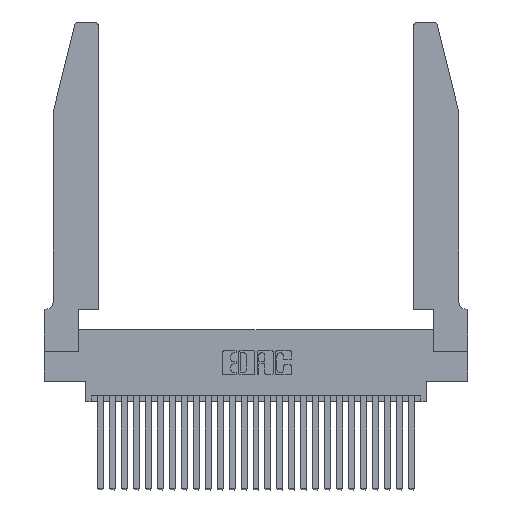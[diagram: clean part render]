
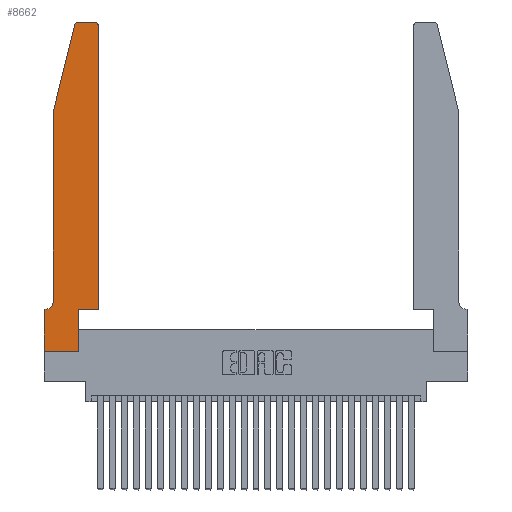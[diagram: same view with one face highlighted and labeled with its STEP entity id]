
A CAD part, top view. The second image highlights one B-rep face of the part: STEP entity #8662.
In plain terms, the highlighted planar face has unit normal (0, 0, 1).
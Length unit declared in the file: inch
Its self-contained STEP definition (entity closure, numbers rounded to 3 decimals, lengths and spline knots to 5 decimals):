
#280 = VECTOR ( 'NONE', #4829, 39.37008 ) ;
#498 = DIRECTION ( 'NONE',  ( 0., 0., 1. ) ) ;
#1354 = LINE ( 'NONE', #3414, #12943 ) ;
#1375 = VERTEX_POINT ( 'NONE', #20350 ) ;
#1484 = EDGE_CURVE ( 'NONE', #25828, #1597, #11867, .T. ) ;
#1553 = VERTEX_POINT ( 'NONE', #9687 ) ;
#1597 = VERTEX_POINT ( 'NONE', #9875 ) ;
#1638 = CARTESIAN_POINT ( 'NONE',  ( 0.4505, 0.35, 0.37 ) ) ;
#1852 = DIRECTION ( 'NONE',  ( 1., 0., 0. ) ) ;
#1901 = CARTESIAN_POINT ( 'NONE',  ( 0.0755, 2., 0.37 ) ) ;
#2112 = LINE ( 'NONE', #6512, #23716 ) ;
#3050 = CARTESIAN_POINT ( 'NONE',  ( 0.0055, 0.35, 0.37 ) ) ;
#3414 = CARTESIAN_POINT ( 'NONE',  ( 0.0755, 2., 0.37 ) ) ;
#3684 = CARTESIAN_POINT ( 'NONE',  ( 0.0755, 0.35, 0.37 ) ) ;
#4137 = CARTESIAN_POINT ( 'NONE',  ( 0., 0., 0.37 ) ) ;
#4829 = DIRECTION ( 'NONE',  ( 0., 1., 0. ) ) ;
#5227 = CIRCLE ( 'NONE', #26367, 0.03 ) ;
#5366 = EDGE_CURVE ( 'NONE', #20245, #25828, #2112, .T. ) ;
#5900 = DIRECTION ( 'NONE',  ( -1., 0., 0. ) ) ;
#6123 = EDGE_CURVE ( 'NONE', #16716, #17226, #22662, .T. ) ;
#6512 = CARTESIAN_POINT ( 'NONE',  ( 0.4505, 0.35, 0.37 ) ) ;
#6935 = AXIS2_PLACEMENT_3D ( 'NONE', #9688, #24693, #11871 ) ;
#7907 = CARTESIAN_POINT ( 'NONE',  ( 0., 0., 0.37 ) ) ;
#8658 = EDGE_CURVE ( 'NONE', #10668, #20245, #23527, .T. ) ;
#8662 = ADVANCED_FACE ( 'NONE', ( #27850 ), #26720, .T. ) ;
#8880 = VECTOR ( 'NONE', #19161, 39.37008 ) ;
#8981 = DIRECTION ( 'NONE',  ( 1., 0., 0. ) ) ;
#9203 = VECTOR ( 'NONE', #5900, 39.37008 ) ;
#9456 = CARTESIAN_POINT ( 'NONE',  ( 0.4205, 2.75, 0.37 ) ) ;
#9627 = EDGE_CURVE ( 'NONE', #17226, #10668, #27796, .T. ) ;
#9687 = CARTESIAN_POINT ( 'NONE',  ( 0.25487, 2.72718, 0.37 ) ) ;
#9688 = CARTESIAN_POINT ( 'NONE',  ( 0., 0.35, 0.37 ) ) ;
#9735 = LINE ( 'NONE', #26990, #21154 ) ;
#9871 = LINE ( 'NONE', #3684, #9203 ) ;
#9875 = CARTESIAN_POINT ( 'NONE',  ( 0.4505, 2.72, 0.37 ) ) ;
#9982 = DIRECTION ( 'NONE',  ( -1., 0., 0. ) ) ;
#10085 = CARTESIAN_POINT ( 'NONE',  ( 0.0755, 0.42, 0.37 ) ) ;
#10401 = CARTESIAN_POINT ( 'NONE',  ( 0.2865, 0., 0.37 ) ) ;
#10472 = ORIENTED_EDGE ( 'NONE', *, *, #17191, .T. ) ;
#10668 = VERTEX_POINT ( 'NONE', #10401 ) ;
#11104 = AXIS2_PLACEMENT_3D ( 'NONE', #13528, #498, #15684 ) ;
#11573 = ORIENTED_EDGE ( 'NONE', *, *, #14667, .T. ) ;
#11858 = ORIENTED_EDGE ( 'NONE', *, *, #18840, .T. ) ;
#11867 = LINE ( 'NONE', #17174, #280 ) ;
#11871 = DIRECTION ( 'NONE',  ( 1., 0., 0. ) ) ;
#12131 = VECTOR ( 'NONE', #22368, 39.37008 ) ;
#12518 = CARTESIAN_POINT ( 'NONE',  ( 0.0055, 0.42, 0.37 ) ) ;
#12870 = DIRECTION ( 'NONE',  ( 1., 0., 0. ) ) ;
#12943 = VECTOR ( 'NONE', #16382, 39.37008 ) ;
#13123 = EDGE_CURVE ( 'NONE', #1597, #21223, #5227, .T. ) ;
#13415 = ORIENTED_EDGE ( 'NONE', *, *, #27085, .T. ) ;
#13528 = CARTESIAN_POINT ( 'NONE',  ( 0.284, 2.72, 0.37 ) ) ;
#13913 = LINE ( 'NONE', #17051, #8880 ) ;
#14460 = EDGE_CURVE ( 'NONE', #1553, #22090, #1354, .T. ) ;
#14667 = EDGE_CURVE ( 'NONE', #22090, #17212, #13913, .T. ) ;
#14668 = DIRECTION ( 'NONE',  ( -1., 0., 0. ) ) ;
#14872 = DIRECTION ( 'NONE',  ( 0., 0., 1. ) ) ;
#15684 = DIRECTION ( 'NONE',  ( 1., 0., 0. ) ) ;
#16100 = CARTESIAN_POINT ( 'NONE',  ( 0.2865, 0.35, 0.37 ) ) ;
#16382 = DIRECTION ( 'NONE',  ( -0.239, -0.971, 0. ) ) ;
#16716 = VERTEX_POINT ( 'NONE', #17163 ) ;
#16811 = AXIS2_PLACEMENT_3D ( 'NONE', #12518, #27446, #14668 ) ;
#17051 = CARTESIAN_POINT ( 'NONE',  ( 0.0755, 2., 0.37 ) ) ;
#17163 = CARTESIAN_POINT ( 'NONE',  ( 0., 0.35, 0.37 ) ) ;
#17174 = CARTESIAN_POINT ( 'NONE',  ( 0.4505, 0.35, 0.37 ) ) ;
#17191 = EDGE_CURVE ( 'NONE', #21223, #1375, #9735, .T. ) ;
#17212 = VERTEX_POINT ( 'NONE', #10085 ) ;
#17226 = VERTEX_POINT ( 'NONE', #7907 ) ;
#18238 = CIRCLE ( 'NONE', #11104, 0.03 ) ;
#18424 = ORIENTED_EDGE ( 'NONE', *, *, #8658, .T. ) ;
#18840 = EDGE_CURVE ( 'NONE', #17212, #19974, #23962, .T. ) ;
#19161 = DIRECTION ( 'NONE',  ( 0., -1., 0. ) ) ;
#19260 = CARTESIAN_POINT ( 'NONE',  ( 0.2865, 0.35, 0.37 ) ) ;
#19974 = VERTEX_POINT ( 'NONE', #3050 ) ;
#20245 = VERTEX_POINT ( 'NONE', #19260 ) ;
#20350 = CARTESIAN_POINT ( 'NONE',  ( 0.284, 2.75, 0.37 ) ) ;
#20771 = ORIENTED_EDGE ( 'NONE', *, *, #27417, .T. ) ;
#21154 = VECTOR ( 'NONE', #9982, 39.37008 ) ;
#21223 = VERTEX_POINT ( 'NONE', #9456 ) ;
#21626 = ORIENTED_EDGE ( 'NONE', *, *, #13123, .T. ) ;
#21695 = ORIENTED_EDGE ( 'NONE', *, *, #1484, .T. ) ;
#22090 = VERTEX_POINT ( 'NONE', #1901 ) ;
#22127 = VECTOR ( 'NONE', #12870, 39.37008 ) ;
#22221 = ORIENTED_EDGE ( 'NONE', *, *, #5366, .T. ) ;
#22243 = CARTESIAN_POINT ( 'NONE',  ( 0., 0., 0.37 ) ) ;
#22368 = DIRECTION ( 'NONE',  ( 0., 1., 0. ) ) ;
#22441 = ORIENTED_EDGE ( 'NONE', *, *, #6123, .T. ) ;
#22662 = LINE ( 'NONE', #22243, #27647 ) ;
#23527 = LINE ( 'NONE', #16100, #12131 ) ;
#23716 = VECTOR ( 'NONE', #8981, 39.37008 ) ;
#23962 = CIRCLE ( 'NONE', #16811, 0.07 ) ;
#24076 = ORIENTED_EDGE ( 'NONE', *, *, #9627, .T. ) ;
#24401 = DIRECTION ( 'NONE',  ( 0., -1., 0. ) ) ;
#24693 = DIRECTION ( 'NONE',  ( 0., 0., 1. ) ) ;
#25828 = VERTEX_POINT ( 'NONE', #1638 ) ;
#26367 = AXIS2_PLACEMENT_3D ( 'NONE', #27644, #14872, #1852 ) ;
#26720 = PLANE ( 'NONE',  #6935 ) ;
#26781 = EDGE_LOOP ( 'NONE', ( #10472, #20771, #27824, #11573, #11858, #13415, #22441, #24076, #18424, #22221, #21695, #21626 ) ) ;
#26990 = CARTESIAN_POINT ( 'NONE',  ( 0.2605, 2.75, 0.37 ) ) ;
#27085 = EDGE_CURVE ( 'NONE', #19974, #16716, #9871, .T. ) ;
#27417 = EDGE_CURVE ( 'NONE', #1375, #1553, #18238, .T. ) ;
#27446 = DIRECTION ( 'NONE',  ( 0., 0., -1. ) ) ;
#27644 = CARTESIAN_POINT ( 'NONE',  ( 0.4205, 2.72, 0.37 ) ) ;
#27647 = VECTOR ( 'NONE', #24401, 39.37008 ) ;
#27796 = LINE ( 'NONE', #4137, #22127 ) ;
#27824 = ORIENTED_EDGE ( 'NONE', *, *, #14460, .T. ) ;
#27850 = FACE_OUTER_BOUND ( 'NONE', #26781, .T. ) ;
